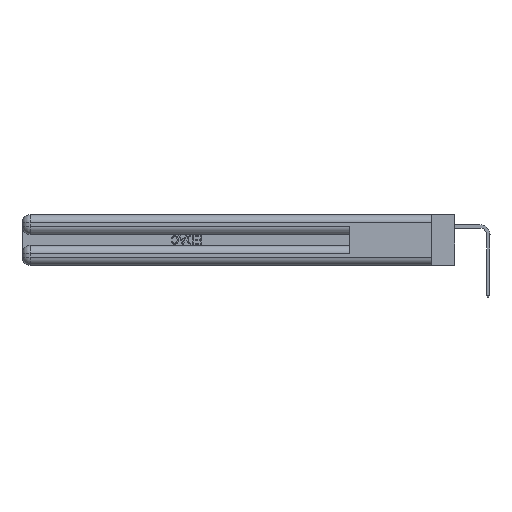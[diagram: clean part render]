
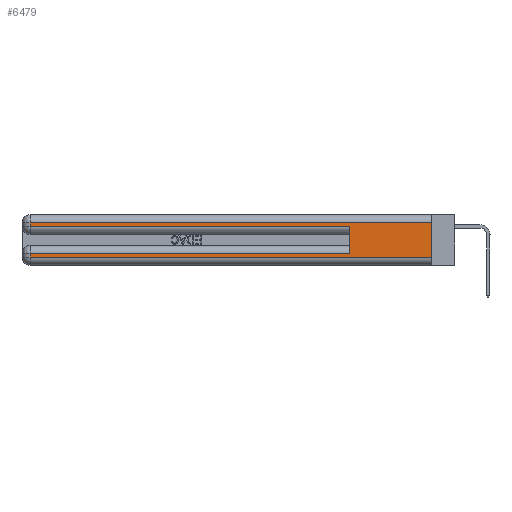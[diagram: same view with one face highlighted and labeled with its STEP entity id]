
A CAD part, left-side view. The second image highlights one B-rep face of the part: STEP entity #6479.
In plain terms, the highlighted planar face has unit normal (-1, 0, 0).
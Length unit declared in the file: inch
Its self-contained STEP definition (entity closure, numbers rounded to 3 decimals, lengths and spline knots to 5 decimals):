
#680 = LINE ( 'NONE', #29713, #31992 ) ;
#3616 = VERTEX_POINT ( 'NONE', #20811 ) ;
#4256 = ORIENTED_EDGE ( 'NONE', *, *, #7875, .T. ) ;
#4282 = FACE_OUTER_BOUND ( 'NONE', #28147, .T. ) ;
#4763 = CARTESIAN_POINT ( 'NONE',  ( 0., 2.94, 0.06 ) ) ;
#6479 = ADVANCED_FACE ( 'NONE', ( #4282 ), #48605, .F. ) ;
#6714 = VECTOR ( 'NONE', #15713, 39.37008 ) ;
#7194 = VERTEX_POINT ( 'NONE', #32482 ) ;
#7875 = EDGE_CURVE ( 'NONE', #40674, #3616, #19738, .T. ) ;
#8591 = VECTOR ( 'NONE', #18559, 39.37008 ) ;
#8741 = VECTOR ( 'NONE', #51565, 39.37008 ) ;
#8809 = VERTEX_POINT ( 'NONE', #34860 ) ;
#8835 = EDGE_CURVE ( 'NONE', #15112, #23394, #29306, .T. ) ;
#9085 = DIRECTION ( 'NONE',  ( 0., 0., 1. ) ) ;
#9619 = VERTEX_POINT ( 'NONE', #48962 ) ;
#10303 = ORIENTED_EDGE ( 'NONE', *, *, #49708, .T. ) ;
#11356 = CARTESIAN_POINT ( 'NONE',  ( 0., 0., 0.37 ) ) ;
#12906 = LINE ( 'NONE', #13609, #43350 ) ;
#13174 = EDGE_CURVE ( 'NONE', #3616, #15112, #14218, .T. ) ;
#13609 = CARTESIAN_POINT ( 'NONE',  ( 0., 2.94, 0.37 ) ) ;
#14218 = LINE ( 'NONE', #45093, #25228 ) ;
#15112 = VERTEX_POINT ( 'NONE', #4763 ) ;
#15713 = DIRECTION ( 'NONE',  ( 0., 0., -1. ) ) ;
#16119 = DIRECTION ( 'NONE',  ( 0., 1., 0. ) ) ;
#17118 = ORIENTED_EDGE ( 'NONE', *, *, #28810, .F. ) ;
#17498 = EDGE_CURVE ( 'NONE', #40674, #39335, #680, .T. ) ;
#18559 = DIRECTION ( 'NONE',  ( 0., -1., 0. ) ) ;
#19071 = LINE ( 'NONE', #19731, #6714 ) ;
#19731 = CARTESIAN_POINT ( 'NONE',  ( 0., 0., 0.37 ) ) ;
#19738 = LINE ( 'NONE', #45044, #50094 ) ;
#19768 = LINE ( 'NONE', #30810, #8741 ) ;
#20243 = ORIENTED_EDGE ( 'NONE', *, *, #24843, .T. ) ;
#20345 = DIRECTION ( 'NONE',  ( 0., 0., -1. ) ) ;
#20810 = EDGE_CURVE ( 'NONE', #7194, #39335, #40100, .T. ) ;
#20811 = CARTESIAN_POINT ( 'NONE',  ( 0., 2.94, 0.085 ) ) ;
#22287 = DIRECTION ( 'NONE',  ( 0., -1., 0. ) ) ;
#22513 = CARTESIAN_POINT ( 'NONE',  ( 0., 0., 0.06 ) ) ;
#23139 = ORIENTED_EDGE ( 'NONE', *, *, #20810, .T. ) ;
#23394 = VERTEX_POINT ( 'NONE', #44707 ) ;
#23831 = DIRECTION ( 'NONE',  ( 1., 0., 0. ) ) ;
#23867 = CARTESIAN_POINT ( 'NONE',  ( 0., 0.6, 0.285 ) ) ;
#24843 = EDGE_CURVE ( 'NONE', #9619, #7194, #12906, .T. ) ;
#25228 = VECTOR ( 'NONE', #20345, 39.37008 ) ;
#26017 = ORIENTED_EDGE ( 'NONE', *, *, #13174, .T. ) ;
#26261 = CARTESIAN_POINT ( 'NONE',  ( 0., 0., 0.285 ) ) ;
#28147 = EDGE_LOOP ( 'NONE', ( #17118, #10303, #20243, #23139, #51929, #4256, #26017, #45984 ) ) ;
#28810 = EDGE_CURVE ( 'NONE', #8809, #23394, #19071, .T. ) ;
#29306 = LINE ( 'NONE', #22513, #8591 ) ;
#29713 = CARTESIAN_POINT ( 'NONE',  ( 0., 0.6, 0.145 ) ) ;
#30810 = CARTESIAN_POINT ( 'NONE',  ( 0., 0., 0.31 ) ) ;
#31992 = VECTOR ( 'NONE', #9085, 39.37008 ) ;
#32431 = AXIS2_PLACEMENT_3D ( 'NONE', #11356, #23831, #52736 ) ;
#32482 = CARTESIAN_POINT ( 'NONE',  ( 0., 2.94, 0.285 ) ) ;
#34860 = CARTESIAN_POINT ( 'NONE',  ( 0., 0., 0.31 ) ) ;
#38799 = VECTOR ( 'NONE', #22287, 39.37008 ) ;
#39335 = VERTEX_POINT ( 'NONE', #23867 ) ;
#40100 = LINE ( 'NONE', #26261, #38799 ) ;
#40674 = VERTEX_POINT ( 'NONE', #44379 ) ;
#43350 = VECTOR ( 'NONE', #46919, 39.37008 ) ;
#44379 = CARTESIAN_POINT ( 'NONE',  ( 0., 0.6, 0.085 ) ) ;
#44707 = CARTESIAN_POINT ( 'NONE',  ( 0., 0., 0.06 ) ) ;
#45044 = CARTESIAN_POINT ( 'NONE',  ( 0., 0., 0.085 ) ) ;
#45093 = CARTESIAN_POINT ( 'NONE',  ( 0., 2.94, 0.37 ) ) ;
#45984 = ORIENTED_EDGE ( 'NONE', *, *, #8835, .T. ) ;
#46919 = DIRECTION ( 'NONE',  ( 0., 0., -1. ) ) ;
#48605 = PLANE ( 'NONE',  #32431 ) ;
#48962 = CARTESIAN_POINT ( 'NONE',  ( 0., 2.94, 0.31 ) ) ;
#49708 = EDGE_CURVE ( 'NONE', #8809, #9619, #19768, .T. ) ;
#50094 = VECTOR ( 'NONE', #16119, 39.37008 ) ;
#51565 = DIRECTION ( 'NONE',  ( 0., 1., 0. ) ) ;
#51929 = ORIENTED_EDGE ( 'NONE', *, *, #17498, .F. ) ;
#52736 = DIRECTION ( 'NONE',  ( 0., 0., -1. ) ) ;
